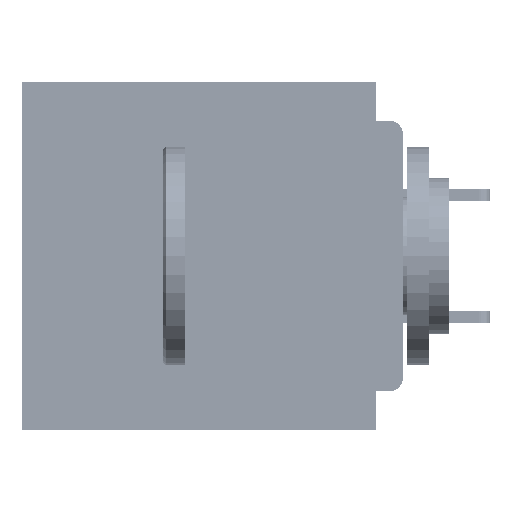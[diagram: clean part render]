
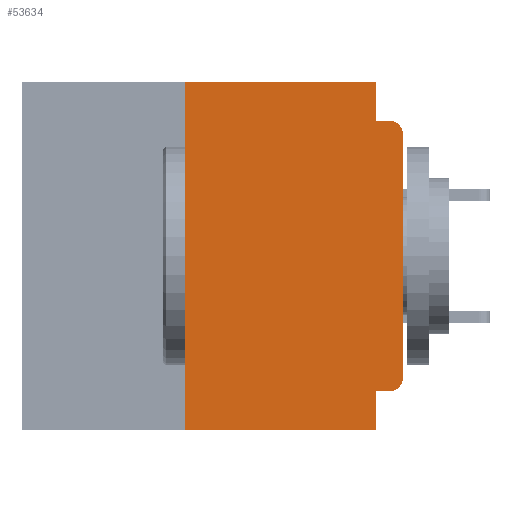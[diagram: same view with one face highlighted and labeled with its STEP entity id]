
A CAD part, left-side view. The second image highlights one B-rep face of the part: STEP entity #53634.
In plain terms, the highlighted planar face has unit normal (-1, 0, 0).
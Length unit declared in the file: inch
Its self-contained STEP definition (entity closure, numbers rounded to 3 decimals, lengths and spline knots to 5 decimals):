
#1107 = VERTEX_POINT ( 'NONE', #35792 ) ;
#1570 = DIRECTION ( 'NONE',  ( 1., 0., 0. ) ) ;
#5621 = VERTEX_POINT ( 'NONE', #17573 ) ;
#5688 = VERTEX_POINT ( 'NONE', #12873 ) ;
#5710 = EDGE_CURVE ( 'NONE', #5688, #44891, #10307, .T. ) ;
#7655 = DIRECTION ( 'NONE',  ( 0., -1., 0. ) ) ;
#10307 = LINE ( 'NONE', #13107, #53824 ) ;
#10803 = ORIENTED_EDGE ( 'NONE', *, *, #63777, .F. ) ;
#11818 = LINE ( 'NONE', #20714, #38159 ) ;
#12538 = CARTESIAN_POINT ( 'NONE',  ( 0., 0.015, -0.355 ) ) ;
#12873 = CARTESIAN_POINT ( 'NONE',  ( 0., 0.031, -0.045 ) ) ;
#13107 = CARTESIAN_POINT ( 'NONE',  ( 0., 0., -0.045 ) ) ;
#13629 = VERTEX_POINT ( 'NONE', #39233 ) ;
#14003 = ORIENTED_EDGE ( 'NONE', *, *, #61415, .F. ) ;
#14109 = VERTEX_POINT ( 'NONE', #16990 ) ;
#14258 = VECTOR ( 'NONE', #7655, 39.37008 ) ;
#15851 = CARTESIAN_POINT ( 'NONE',  ( 0., 0.437, -0.4 ) ) ;
#16990 = CARTESIAN_POINT ( 'NONE',  ( 0., 0.031, -0.355 ) ) ;
#17573 = CARTESIAN_POINT ( 'NONE',  ( 0., 0., -0.06 ) ) ;
#18497 = CARTESIAN_POINT ( 'NONE',  ( 0., 0.015, -0.34 ) ) ;
#20714 = CARTESIAN_POINT ( 'NONE',  ( 0., 0., -0.355 ) ) ;
#20960 = LINE ( 'NONE', #60071, #56138 ) ;
#22060 = EDGE_CURVE ( 'NONE', #39867, #14109, #11818, .T. ) ;
#22192 = CIRCLE ( 'NONE', #30279, 0.015 ) ;
#22872 = DIRECTION ( 'NONE',  ( 0., 0., 1. ) ) ;
#23779 = DIRECTION ( 'NONE',  ( 0., -1., 0. ) ) ;
#23786 = DIRECTION ( 'NONE',  ( 0., 0., -1. ) ) ;
#24845 = DIRECTION ( 'NONE',  ( -1., 0., 0. ) ) ;
#25842 = EDGE_CURVE ( 'NONE', #66168, #26631, #46196, .T. ) ;
#25984 = DIRECTION ( 'NONE',  ( 0., 1., 0. ) ) ;
#26631 = VERTEX_POINT ( 'NONE', #38214 ) ;
#27789 = VECTOR ( 'NONE', #60842, 39.37008 ) ;
#29067 = ORIENTED_EDGE ( 'NONE', *, *, #34962, .T. ) ;
#30279 = AXIS2_PLACEMENT_3D ( 'NONE', #56163, #24845, #61445 ) ;
#30636 = ORIENTED_EDGE ( 'NONE', *, *, #48306, .T. ) ;
#31935 = VECTOR ( 'NONE', #63687, 39.37008 ) ;
#33143 = CARTESIAN_POINT ( 'NONE',  ( 0., 0., 0. ) ) ;
#33198 = PLANE ( 'NONE',  #65243 ) ;
#33970 = DIRECTION ( 'NONE',  ( 0., 0., 1. ) ) ;
#34962 = EDGE_CURVE ( 'NONE', #5621, #44891, #22192, .T. ) ;
#35248 = EDGE_CURVE ( 'NONE', #14109, #26631, #45827, .T. ) ;
#35792 = CARTESIAN_POINT ( 'NONE',  ( 0., 0.031, 0. ) ) ;
#37752 = CARTESIAN_POINT ( 'NONE',  ( 0., 0.25, -0.4 ) ) ;
#38159 = VECTOR ( 'NONE', #25984, 39.37008 ) ;
#38214 = CARTESIAN_POINT ( 'NONE',  ( 0., 0.031, -0.4 ) ) ;
#38454 = DIRECTION ( 'NONE',  ( 0., 0., -1. ) ) ;
#39233 = CARTESIAN_POINT ( 'NONE',  ( 0., 0., -0.34 ) ) ;
#39679 = FACE_OUTER_BOUND ( 'NONE', #52488, .T. ) ;
#39867 = VERTEX_POINT ( 'NONE', #12538 ) ;
#40381 = AXIS2_PLACEMENT_3D ( 'NONE', #18497, #55069, #23786 ) ;
#40503 = LINE ( 'NONE', #65249, #14258 ) ;
#43294 = LINE ( 'NONE', #66068, #27789 ) ;
#44891 = VERTEX_POINT ( 'NONE', #56736 ) ;
#45827 = LINE ( 'NONE', #63231, #31935 ) ;
#46147 = CARTESIAN_POINT ( 'NONE',  ( 0., 0.25, 0. ) ) ;
#46196 = LINE ( 'NONE', #15851, #60146 ) ;
#47616 = ORIENTED_EDGE ( 'NONE', *, *, #5710, .F. ) ;
#48306 = EDGE_CURVE ( 'NONE', #13629, #5621, #49457, .T. ) ;
#49457 = LINE ( 'NONE', #33143, #61799 ) ;
#52488 = EDGE_LOOP ( 'NONE', ( #30636, #29067, #47616, #14003, #10803, #66429, #59183, #54253, #57338, #55298 ) ) ;
#53634 = ADVANCED_FACE ( 'NONE', ( #39679 ), #33198, .F. ) ;
#53824 = VECTOR ( 'NONE', #23779, 39.37008 ) ;
#54253 = ORIENTED_EDGE ( 'NONE', *, *, #35248, .F. ) ;
#55069 = DIRECTION ( 'NONE',  ( -1., 0., 0. ) ) ;
#55298 = ORIENTED_EDGE ( 'NONE', *, *, #56681, .T. ) ;
#56138 = VECTOR ( 'NONE', #33970, 39.37008 ) ;
#56163 = CARTESIAN_POINT ( 'NONE',  ( 0., 0.015, -0.06 ) ) ;
#56681 = EDGE_CURVE ( 'NONE', #39867, #13629, #62316, .T. ) ;
#56736 = CARTESIAN_POINT ( 'NONE',  ( 0., 0.015, -0.045 ) ) ;
#57338 = ORIENTED_EDGE ( 'NONE', *, *, #22060, .F. ) ;
#59183 = ORIENTED_EDGE ( 'NONE', *, *, #25842, .T. ) ;
#59301 = CARTESIAN_POINT ( 'NONE',  ( 0., 0.437, 0. ) ) ;
#60071 = CARTESIAN_POINT ( 'NONE',  ( 0., 0.25, -0.4 ) ) ;
#60146 = VECTOR ( 'NONE', #62803, 39.37008 ) ;
#60842 = DIRECTION ( 'NONE',  ( 0., 0., -1. ) ) ;
#61415 = EDGE_CURVE ( 'NONE', #1107, #5688, #43294, .T. ) ;
#61445 = DIRECTION ( 'NONE',  ( 0., 0., -1. ) ) ;
#61799 = VECTOR ( 'NONE', #22872, 39.37008 ) ;
#62316 = CIRCLE ( 'NONE', #40381, 0.015 ) ;
#62803 = DIRECTION ( 'NONE',  ( 0., -1., 0. ) ) ;
#62882 = VERTEX_POINT ( 'NONE', #46147 ) ;
#63231 = CARTESIAN_POINT ( 'NONE',  ( 0., 0.031, -0.4 ) ) ;
#63292 = EDGE_CURVE ( 'NONE', #66168, #62882, #20960, .T. ) ;
#63687 = DIRECTION ( 'NONE',  ( 0., 0., -1. ) ) ;
#63777 = EDGE_CURVE ( 'NONE', #62882, #1107, #40503, .T. ) ;
#65243 = AXIS2_PLACEMENT_3D ( 'NONE', #59301, #1570, #38454 ) ;
#65249 = CARTESIAN_POINT ( 'NONE',  ( 0., 0.437, 0. ) ) ;
#66068 = CARTESIAN_POINT ( 'NONE',  ( 0., 0.031, 0. ) ) ;
#66168 = VERTEX_POINT ( 'NONE', #37752 ) ;
#66429 = ORIENTED_EDGE ( 'NONE', *, *, #63292, .F. ) ;
